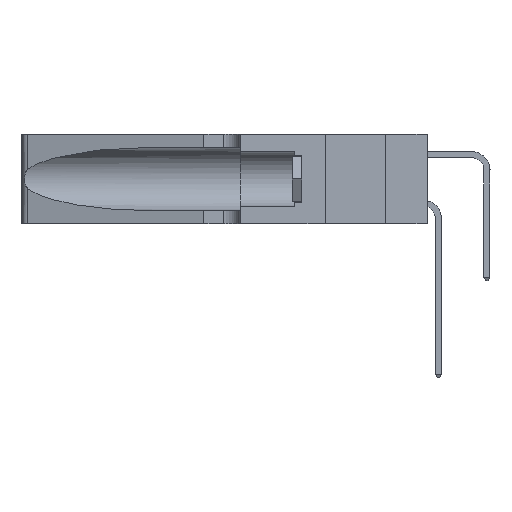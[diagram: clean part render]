
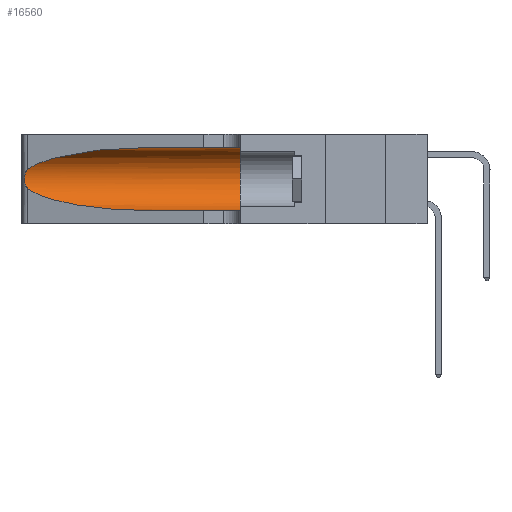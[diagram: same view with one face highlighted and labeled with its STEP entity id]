
A CAD part, left-side view. The second image highlights one B-rep face of the part: STEP entity #16560.
In plain terms, the highlighted cylindrical face has radius 3.308 mm (diameter 6.617 mm), a partial arc.
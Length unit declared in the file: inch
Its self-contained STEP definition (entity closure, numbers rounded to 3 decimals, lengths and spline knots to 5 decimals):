
#243 = LINE ( 'NONE', #27448, #27133 ) ;
#259 =( BOUNDED_CURVE ( )  B_SPLINE_CURVE ( 3, ( #16590, #11532, #6545, #32338 ),
 .UNSPECIFIED., .F., .T. ) 
 B_SPLINE_CURVE_WITH_KNOTS ( ( 4, 4 ),
 ( 3.44316, 4.71239 ),
 .UNSPECIFIED. ) 
 CURVE ( )  GEOMETRIC_REPRESENTATION_ITEM ( )  RATIONAL_B_SPLINE_CURVE ( ( 1., 0.87, 0.87, 1. ) ) 
 REPRESENTATION_ITEM ( '' )  );
#370 = CARTESIAN_POINT ( 'NONE',  ( 0.26075, 1.23896, 0.19203 ) ) ;
#395 = LINE ( 'NONE', #20073, #26478 ) ;
#421 = VERTEX_POINT ( 'NONE', #27615 ) ;
#423 = DIRECTION ( 'NONE',  ( 0., 1., 0. ) ) ;
#1233 = EDGE_CURVE ( 'NONE', #5156, #6926, #259, .T. ) ;
#1282 = FACE_OUTER_BOUND ( 'NONE', #7082, .T. ) ;
#1713 = EDGE_CURVE ( 'NONE', #29035, #10895, #2415, .T. ) ;
#2312 = ORIENTED_EDGE ( 'NONE', *, *, #1713, .F. ) ;
#2415 = CIRCLE ( 'NONE', #18931, 0.13025 ) ;
#2531 = CARTESIAN_POINT ( 'NONE',  ( 0.25487, 1.22718, 0.22369 ) ) ;
#2606 = CARTESIAN_POINT ( 'NONE',  ( 0.25787, 1.23484, 0.2124 ) ) ;
#4704 = ORIENTED_EDGE ( 'NONE', *, *, #23554, .T. ) ;
#5156 = VERTEX_POINT ( 'NONE', #19212 ) ;
#5723 = CARTESIAN_POINT ( 'NONE',  ( 0.18966, 0.96281, 0.31525 ) ) ;
#5862 = CARTESIAN_POINT ( 'NONE',  ( 0.26075, 1.23896, 0.178 ) ) ;
#6545 = CARTESIAN_POINT ( 'NONE',  ( 0.18966, 0.96281, 0.05475 ) ) ;
#6674 = ORIENTED_EDGE ( 'NONE', *, *, #28925, .T. ) ;
#6926 = VERTEX_POINT ( 'NONE', #27466 ) ;
#7082 = EDGE_LOOP ( 'NONE', ( #6674, #10279, #11352, #4704, #2312, #31325 ) ) ;
#8494 = CARTESIAN_POINT ( 'NONE',  ( 0.25856, 1.23593, 0.16098 ) ) ;
#8899 = CARTESIAN_POINT ( 'NONE',  ( 0.1305, 0.35, 0.31525 ) ) ;
#10238 = CARTESIAN_POINT ( 'NONE',  ( 0.25555, 1.22994, 0.2215 ) ) ;
#10279 = ORIENTED_EDGE ( 'NONE', *, *, #25254, .T. ) ;
#10895 = VERTEX_POINT ( 'NONE', #33483 ) ;
#11352 = ORIENTED_EDGE ( 'NONE', *, *, #1233, .T. ) ;
#11379 = CARTESIAN_POINT ( 'NONE',  ( 0.25639, 1.23184, 0.21858 ) ) ;
#11532 = CARTESIAN_POINT ( 'NONE',  ( 0.2373, 1.15595, 0.08982 ) ) ;
#12249 = CARTESIAN_POINT ( 'NONE',  ( 0.25487, 1.22718, 0.14631 ) ) ;
#12465 = DIRECTION ( 'NONE',  ( 0., -1., 0. ) ) ;
#13088 = CARTESIAN_POINT ( 'NONE',  ( 0.25854, 1.2359, 0.20912 ) ) ;
#15060 = DIRECTION ( 'NONE',  ( 0., -1., 0. ) ) ;
#16380 = CARTESIAN_POINT ( 'NONE',  ( 0.25789, 1.23486, 0.15765 ) ) ;
#16560 = ADVANCED_FACE ( 'NONE', ( #1282 ), #32230, .F. ) ;
#16590 = CARTESIAN_POINT ( 'NONE',  ( 0.25487, 1.22718, 0.14631 ) ) ;
#17685 = DIRECTION ( 'NONE',  ( 0., 0., -1. ) ) ;
#18931 = AXIS2_PLACEMENT_3D ( 'NONE', #33365, #423, #19737 ) ;
#19212 = CARTESIAN_POINT ( 'NONE',  ( 0.25487, 1.22718, 0.14631 ) ) ;
#19737 = DIRECTION ( 'NONE',  ( 0., 0., 1. ) ) ;
#20073 = CARTESIAN_POINT ( 'NONE',  ( 0.1305, 1.61858, 0.31525 ) ) ;
#20882 = AXIS2_PLACEMENT_3D ( 'NONE', #25601, #12465, #17685 ) ;
#20990 = B_SPLINE_CURVE_WITH_KNOTS ( 'NONE', 3,
 ( #27846, #10238, #11379, #2606, #13088, #31888, #370, #5862, #24065, #8494, #16380, #25060, #24823, #12249 ),
 .UNSPECIFIED., .F., .F.,
 ( 4, 2, 2, 2, 2, 2, 4 ),
 ( 0., 0.00027, 0.00053, 0.00107, 0.0016, 0.00187, 0.00214 ),
 .UNSPECIFIED. ) ;
#21451 = CARTESIAN_POINT ( 'NONE',  ( 0.2373, 1.15595, 0.28018 ) ) ;
#22020 =( BOUNDED_CURVE ( )  B_SPLINE_CURVE ( 3, ( #29159, #5723, #21451, #31522 ),
 .UNSPECIFIED., .F., .F. ) 
 B_SPLINE_CURVE_WITH_KNOTS ( ( 4, 4 ),
 ( 1.5708, 2.84003 ),
 .UNSPECIFIED. ) 
 CURVE ( )  GEOMETRIC_REPRESENTATION_ITEM ( )  RATIONAL_B_SPLINE_CURVE ( ( 1., 0.87, 0.87, 1. ) ) 
 REPRESENTATION_ITEM ( '' )  );
#23554 = EDGE_CURVE ( 'NONE', #6926, #10895, #243, .T. ) ;
#24065 = CARTESIAN_POINT ( 'NONE',  ( 0.26017, 1.23833, 0.17102 ) ) ;
#24823 = CARTESIAN_POINT ( 'NONE',  ( 0.25555, 1.22993, 0.14849 ) ) ;
#25060 = CARTESIAN_POINT ( 'NONE',  ( 0.25639, 1.23186, 0.15144 ) ) ;
#25254 = EDGE_CURVE ( 'NONE', #25294, #5156, #20990, .T. ) ;
#25294 = VERTEX_POINT ( 'NONE', #2531 ) ;
#25601 = CARTESIAN_POINT ( 'NONE',  ( 0.1305, 1.61858, 0.185 ) ) ;
#26478 = VECTOR ( 'NONE', #15060, 39.37008 ) ;
#27133 = VECTOR ( 'NONE', #27556, 39.37008 ) ;
#27448 = CARTESIAN_POINT ( 'NONE',  ( 0.1305, 1.61858, 0.05475 ) ) ;
#27466 = CARTESIAN_POINT ( 'NONE',  ( 0.1305, 0.72297, 0.05475 ) ) ;
#27556 = DIRECTION ( 'NONE',  ( 0., -1., 0. ) ) ;
#27615 = CARTESIAN_POINT ( 'NONE',  ( 0.1305, 0.72297, 0.31525 ) ) ;
#27846 = CARTESIAN_POINT ( 'NONE',  ( 0.25487, 1.22718, 0.22369 ) ) ;
#28925 = EDGE_CURVE ( 'NONE', #421, #25294, #22020, .T. ) ;
#29035 = VERTEX_POINT ( 'NONE', #8899 ) ;
#29159 = CARTESIAN_POINT ( 'NONE',  ( 0.1305, 0.72297, 0.31525 ) ) ;
#31325 = ORIENTED_EDGE ( 'NONE', *, *, #32742, .F. ) ;
#31522 = CARTESIAN_POINT ( 'NONE',  ( 0.25487, 1.22718, 0.22369 ) ) ;
#31888 = CARTESIAN_POINT ( 'NONE',  ( 0.26018, 1.23835, 0.19895 ) ) ;
#32230 = CYLINDRICAL_SURFACE ( 'NONE', #20882, 0.13025 ) ;
#32338 = CARTESIAN_POINT ( 'NONE',  ( 0.1305, 0.72297, 0.05475 ) ) ;
#32742 = EDGE_CURVE ( 'NONE', #421, #29035, #395, .T. ) ;
#33365 = CARTESIAN_POINT ( 'NONE',  ( 0.1305, 0.35, 0.185 ) ) ;
#33483 = CARTESIAN_POINT ( 'NONE',  ( 0.1305, 0.35, 0.05475 ) ) ;
